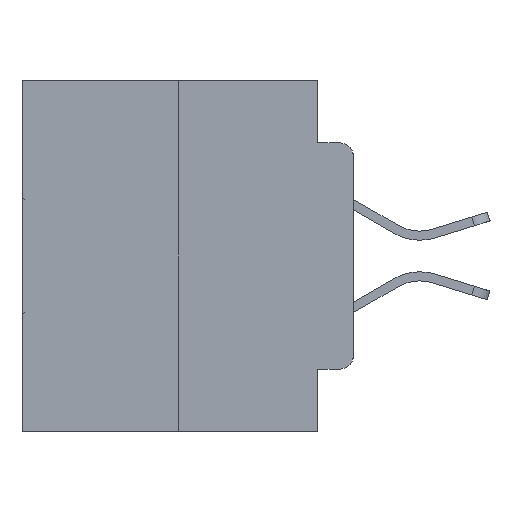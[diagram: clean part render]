
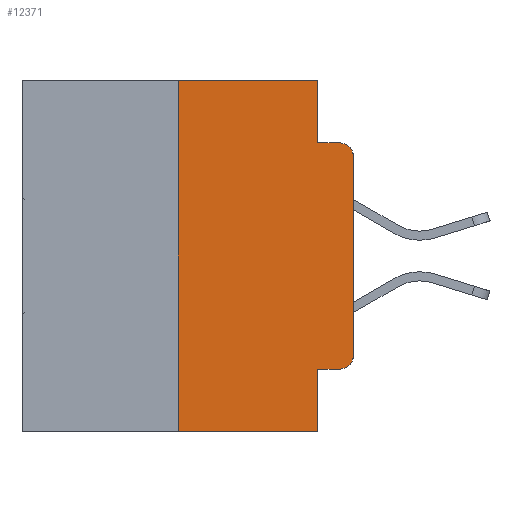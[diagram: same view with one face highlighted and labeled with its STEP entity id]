
A CAD part, left-side view. The second image highlights one B-rep face of the part: STEP entity #12371.
In plain terms, the highlighted planar face has unit normal (-1, 0, 0).
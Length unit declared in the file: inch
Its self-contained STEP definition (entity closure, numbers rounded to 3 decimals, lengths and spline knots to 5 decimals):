
#10 = CARTESIAN_POINT ( 'NONE',  ( 0., 0.051, 0. ) ) ;
#291 = ORIENTED_EDGE ( 'NONE', *, *, #24320, .F. ) ;
#301 = EDGE_CURVE ( 'NONE', #11217, #7319, #13007, .T. ) ;
#505 = CARTESIAN_POINT ( 'NONE',  ( 0., 0.051, 0. ) ) ;
#514 = VERTEX_POINT ( 'NONE', #24754 ) ;
#751 = CARTESIAN_POINT ( 'NONE',  ( 0., 0.473, 0. ) ) ;
#788 = DIRECTION ( 'NONE',  ( -1., 0., 0. ) ) ;
#795 = VECTOR ( 'NONE', #13740, 39.37008 ) ;
#921 = CARTESIAN_POINT ( 'NONE',  ( 0., 0., 0. ) ) ;
#1741 = CARTESIAN_POINT ( 'NONE',  ( 0., 0.02, -0.3915 ) ) ;
#2246 = EDGE_CURVE ( 'NONE', #25292, #514, #15968, .T. ) ;
#4113 = VECTOR ( 'NONE', #20841, 39.37008 ) ;
#4224 = VECTOR ( 'NONE', #13584, 39.37008 ) ;
#4347 = VECTOR ( 'NONE', #28134, 39.37008 ) ;
#5060 = LINE ( 'NONE', #12986, #4347 ) ;
#5227 = AXIS2_PLACEMENT_3D ( 'NONE', #751, #9913, #25169 ) ;
#5234 = VECTOR ( 'NONE', #17518, 39.37008 ) ;
#5429 = AXIS2_PLACEMENT_3D ( 'NONE', #25049, #12029, #27205 ) ;
#5926 = VERTEX_POINT ( 'NONE', #505 ) ;
#6029 = EDGE_CURVE ( 'NONE', #7319, #12467, #20253, .T. ) ;
#6213 = DIRECTION ( 'NONE',  ( 0., -1., 0. ) ) ;
#7319 = VERTEX_POINT ( 'NONE', #21021 ) ;
#8006 = VECTOR ( 'NONE', #9777, 39.37008 ) ;
#8546 = VECTOR ( 'NONE', #14395, 39.37008 ) ;
#8714 = LINE ( 'NONE', #16404, #8006 ) ;
#9600 = CARTESIAN_POINT ( 'NONE',  ( 0., 0.25, 0. ) ) ;
#9777 = DIRECTION ( 'NONE',  ( 0., -1., 0. ) ) ;
#9913 = DIRECTION ( 'NONE',  ( 1., 0., 0. ) ) ;
#9941 = CARTESIAN_POINT ( 'NONE',  ( 0., 0.051, -0.0885 ) ) ;
#10227 = EDGE_CURVE ( 'NONE', #5926, #25292, #23730, .T. ) ;
#10821 = VERTEX_POINT ( 'NONE', #10870 ) ;
#10870 = CARTESIAN_POINT ( 'NONE',  ( 0., 0.051, -0.4115 ) ) ;
#11217 = VERTEX_POINT ( 'NONE', #16870 ) ;
#11339 = ORIENTED_EDGE ( 'NONE', *, *, #13976, .T. ) ;
#11959 = ORIENTED_EDGE ( 'NONE', *, *, #15664, .F. ) ;
#12029 = DIRECTION ( 'NONE',  ( -1., 0., 0. ) ) ;
#12371 = ADVANCED_FACE ( 'NONE', ( #12687 ), #23028, .F. ) ;
#12467 = VERTEX_POINT ( 'NONE', #14611 ) ;
#12643 = VECTOR ( 'NONE', #6213, 39.37008 ) ;
#12687 = FACE_OUTER_BOUND ( 'NONE', #15576, .T. ) ;
#12986 = CARTESIAN_POINT ( 'NONE',  ( 0., 0.25, 0. ) ) ;
#13007 = CIRCLE ( 'NONE', #19347, 0.02 ) ;
#13584 = DIRECTION ( 'NONE',  ( 0., 0., -1. ) ) ;
#13587 = ORIENTED_EDGE ( 'NONE', *, *, #6029, .T. ) ;
#13740 = DIRECTION ( 'NONE',  ( 0., 0., -1. ) ) ;
#13976 = EDGE_CURVE ( 'NONE', #22504, #22663, #24227, .T. ) ;
#14005 = ORIENTED_EDGE ( 'NONE', *, *, #28076, .F. ) ;
#14395 = DIRECTION ( 'NONE',  ( 0., 0., 1. ) ) ;
#14611 = CARTESIAN_POINT ( 'NONE',  ( 0., 0., -0.1085 ) ) ;
#15474 = CARTESIAN_POINT ( 'NONE',  ( 0., 0.25, -0.5 ) ) ;
#15576 = EDGE_LOOP ( 'NONE', ( #13587, #21830, #23173, #27900, #11959, #14005, #11339, #291, #24628, #15832 ) ) ;
#15664 = EDGE_CURVE ( 'NONE', #25780, #5926, #8714, .T. ) ;
#15832 = ORIENTED_EDGE ( 'NONE', *, *, #301, .T. ) ;
#15968 = LINE ( 'NONE', #18222, #4113 ) ;
#16033 = CARTESIAN_POINT ( 'NONE',  ( 0., 0.051, -0.5 ) ) ;
#16063 = LINE ( 'NONE', #10, #4224 ) ;
#16404 = CARTESIAN_POINT ( 'NONE',  ( 0., 0.473, 0. ) ) ;
#16870 = CARTESIAN_POINT ( 'NONE',  ( 0., 0.02, -0.4115 ) ) ;
#17518 = DIRECTION ( 'NONE',  ( 0., -1., 0. ) ) ;
#17750 = CIRCLE ( 'NONE', #5429, 0.02 ) ;
#18165 = EDGE_CURVE ( 'NONE', #10821, #11217, #23516, .T. ) ;
#18222 = CARTESIAN_POINT ( 'NONE',  ( 0., 0.051, -0.0885 ) ) ;
#19347 = AXIS2_PLACEMENT_3D ( 'NONE', #1741, #788, #24064 ) ;
#19470 = CARTESIAN_POINT ( 'NONE',  ( 0., 0.473, -0.5 ) ) ;
#19752 = CARTESIAN_POINT ( 'NONE',  ( 0., 0.051, -0.4115 ) ) ;
#20233 = CARTESIAN_POINT ( 'NONE',  ( 0., 0.051, 0. ) ) ;
#20253 = LINE ( 'NONE', #921, #8546 ) ;
#20841 = DIRECTION ( 'NONE',  ( 0., -1., 0. ) ) ;
#21021 = CARTESIAN_POINT ( 'NONE',  ( 0., 0., -0.3915 ) ) ;
#21830 = ORIENTED_EDGE ( 'NONE', *, *, #24484, .T. ) ;
#22504 = VERTEX_POINT ( 'NONE', #15474 ) ;
#22663 = VERTEX_POINT ( 'NONE', #16033 ) ;
#23028 = PLANE ( 'NONE',  #5227 ) ;
#23173 = ORIENTED_EDGE ( 'NONE', *, *, #2246, .F. ) ;
#23516 = LINE ( 'NONE', #19752, #5234 ) ;
#23730 = LINE ( 'NONE', #20233, #795 ) ;
#24064 = DIRECTION ( 'NONE',  ( 0., 0., -1. ) ) ;
#24227 = LINE ( 'NONE', #19470, #12643 ) ;
#24320 = EDGE_CURVE ( 'NONE', #10821, #22663, #16063, .T. ) ;
#24484 = EDGE_CURVE ( 'NONE', #12467, #514, #17750, .T. ) ;
#24628 = ORIENTED_EDGE ( 'NONE', *, *, #18165, .T. ) ;
#24754 = CARTESIAN_POINT ( 'NONE',  ( 0., 0.02, -0.0885 ) ) ;
#25049 = CARTESIAN_POINT ( 'NONE',  ( 0., 0.02, -0.1085 ) ) ;
#25169 = DIRECTION ( 'NONE',  ( 0., 0., -1. ) ) ;
#25292 = VERTEX_POINT ( 'NONE', #9941 ) ;
#25780 = VERTEX_POINT ( 'NONE', #9600 ) ;
#27205 = DIRECTION ( 'NONE',  ( 0., 0., -1. ) ) ;
#27900 = ORIENTED_EDGE ( 'NONE', *, *, #10227, .F. ) ;
#28076 = EDGE_CURVE ( 'NONE', #22504, #25780, #5060, .T. ) ;
#28134 = DIRECTION ( 'NONE',  ( 0., 0., 1. ) ) ;
